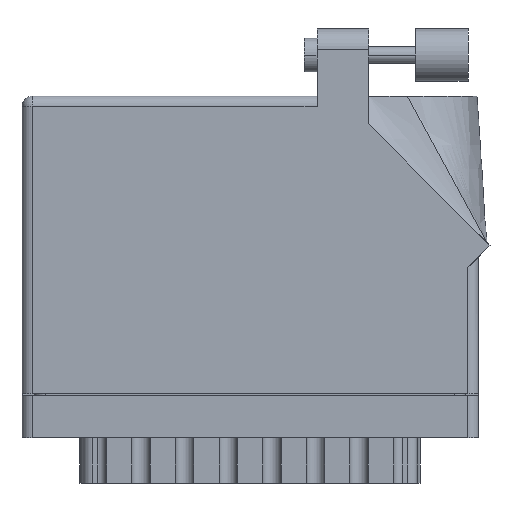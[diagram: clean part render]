
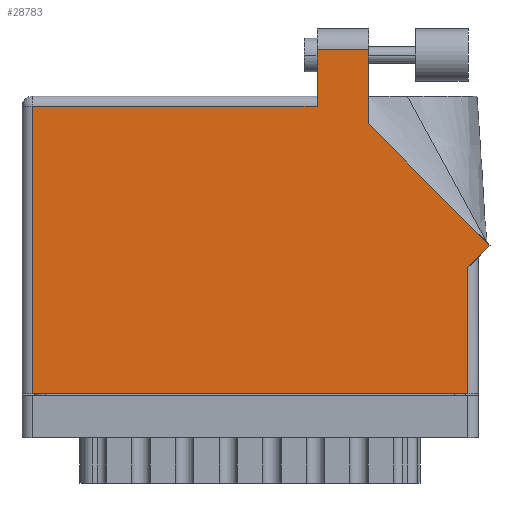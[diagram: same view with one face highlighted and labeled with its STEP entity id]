
A CAD part, front view. The second image highlights one B-rep face of the part: STEP entity #28783.
In plain terms, the highlighted face is planar.
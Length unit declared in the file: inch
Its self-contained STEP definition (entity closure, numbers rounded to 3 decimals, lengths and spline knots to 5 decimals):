
#1003 = DIRECTION ( 'NONE',  ( 0.707, 0.707, 0. ) ) ;
#2508 = ORIENTED_EDGE ( 'NONE', *, *, #10606, .T. ) ;
#4275 = CARTESIAN_POINT ( 'NONE',  ( 2.78871, 0.88571, 0. ) ) ;
#4432 = LINE ( 'NONE', #39975, #25577 ) ;
#4710 = VECTOR ( 'NONE', #21196, 39.37008 ) ;
#4968 = DIRECTION ( 'NONE',  ( 0., -1., 0. ) ) ;
#5135 = LINE ( 'NONE', #36905, #26316 ) ;
#5680 = ORIENTED_EDGE ( 'NONE', *, *, #43925, .T. ) ;
#6126 = LINE ( 'NONE', #54887, #30542 ) ;
#8485 = VERTEX_POINT ( 'NONE', #66346 ) ;
#8774 = LINE ( 'NONE', #14644, #66543 ) ;
#9948 = EDGE_CURVE ( 'NONE', #45223, #14900, #4432, .T. ) ;
#10449 = LINE ( 'NONE', #15242, #34849 ) ;
#10606 = EDGE_CURVE ( 'NONE', #60431, #51326, #5135, .T. ) ;
#11034 = CARTESIAN_POINT ( 'NONE',  ( 2.718, 0.815, 0. ) ) ;
#14378 = LINE ( 'NONE', #4275, #53429 ) ;
#14506 = LINE ( 'NONE', #11034, #49414 ) ;
#14644 = CARTESIAN_POINT ( 'NONE',  ( 2.656, 0.815, 0. ) ) ;
#14900 = VERTEX_POINT ( 'NONE', #62461 ) ;
#15081 = VECTOR ( 'NONE', #45955, 39.37008 ) ;
#15198 = DIRECTION ( 'NONE',  ( 0., 0., -1. ) ) ;
#15242 = CARTESIAN_POINT ( 'NONE',  ( 1.758, 1.775, 0. ) ) ;
#15254 = EDGE_LOOP ( 'NONE', ( #42660, #59265, #28161, #42583, #2508, #37288, #5680, #33372, #50235 ) ) ;
#15649 = EDGE_CURVE ( 'NONE', #51323, #59387, #14506, .T. ) ;
#17108 = EDGE_CURVE ( 'NONE', #51326, #8485, #26468, .T. ) ;
#18757 = CARTESIAN_POINT ( 'NONE',  ( 2.656, 0.753, 0. ) ) ;
#21196 = DIRECTION ( 'NONE',  ( 0., 1., 0. ) ) ;
#22940 = VERTEX_POINT ( 'NONE', #36296 ) ;
#23901 = EDGE_CURVE ( 'NONE', #14900, #54092, #10449, .T. ) ;
#25178 = DIRECTION ( 'NONE',  ( -1., 0., 0. ) ) ;
#25197 = DIRECTION ( 'NONE',  ( -0.707, 0.707, 0. ) ) ;
#25412 = PLANE ( 'NONE',  #38828 ) ;
#25577 = VECTOR ( 'NONE', #36327, 39.37008 ) ;
#26316 = VECTOR ( 'NONE', #58099, 39.37008 ) ;
#26468 = LINE ( 'NONE', #40955, #15081 ) ;
#26677 = CARTESIAN_POINT ( 'NONE',  ( 2.065, 1.60942, 0. ) ) ;
#28161 = ORIENTED_EDGE ( 'NONE', *, *, #23901, .T. ) ;
#28783 = ADVANCED_FACE ( 'NONE', ( #59992 ), #25412, .F. ) ;
#29410 = EDGE_CURVE ( 'NONE', #59387, #22940, #14378, .T. ) ;
#30542 = VECTOR ( 'NONE', #39836, 39.37008 ) ;
#33372 = ORIENTED_EDGE ( 'NONE', *, *, #15649, .T. ) ;
#34849 = VECTOR ( 'NONE', #4968, 39.37008 ) ;
#35710 = DIRECTION ( 'NONE',  ( 0., 1., 0. ) ) ;
#36296 = CARTESIAN_POINT ( 'NONE',  ( 2.065, 1.60942, 0. ) ) ;
#36327 = DIRECTION ( 'NONE',  ( -1., 0., 0. ) ) ;
#36905 = CARTESIAN_POINT ( 'NONE',  ( 0.062, 0., 0. ) ) ;
#37288 = ORIENTED_EDGE ( 'NONE', *, *, #17108, .T. ) ;
#37952 = CARTESIAN_POINT ( 'NONE',  ( 1.758, 1.713, 0. ) ) ;
#38828 = AXIS2_PLACEMENT_3D ( 'NONE', #66929, #15198, #25178 ) ;
#39836 = DIRECTION ( 'NONE',  ( -1., 0., 0. ) ) ;
#39975 = CARTESIAN_POINT ( 'NONE',  ( 1.758, 2.05, 0. ) ) ;
#40955 = CARTESIAN_POINT ( 'NONE',  ( 0., 0., 0. ) ) ;
#42583 = ORIENTED_EDGE ( 'NONE', *, *, #45388, .T. ) ;
#42660 = ORIENTED_EDGE ( 'NONE', *, *, #67329, .T. ) ;
#43925 = EDGE_CURVE ( 'NONE', #8485, #51323, #8774, .T. ) ;
#45223 = VERTEX_POINT ( 'NONE', #48953 ) ;
#45388 = EDGE_CURVE ( 'NONE', #54092, #60431, #6126, .T. ) ;
#45955 = DIRECTION ( 'NONE',  ( 1., 0., 0. ) ) ;
#48522 = CARTESIAN_POINT ( 'NONE',  ( 2.78871, 0.88571, 0. ) ) ;
#48953 = CARTESIAN_POINT ( 'NONE',  ( 2.065, 2.05, 0. ) ) ;
#49414 = VECTOR ( 'NONE', #1003, 39.37008 ) ;
#50235 = ORIENTED_EDGE ( 'NONE', *, *, #29410, .T. ) ;
#51323 = VERTEX_POINT ( 'NONE', #18757 ) ;
#51326 = VERTEX_POINT ( 'NONE', #66227 ) ;
#53429 = VECTOR ( 'NONE', #25197, 39.37008 ) ;
#54092 = VERTEX_POINT ( 'NONE', #37952 ) ;
#54887 = CARTESIAN_POINT ( 'NONE',  ( 0., 1.713, 0. ) ) ;
#56705 = CARTESIAN_POINT ( 'NONE',  ( 0.062, 1.713, 0. ) ) ;
#58099 = DIRECTION ( 'NONE',  ( 0., -1., 0. ) ) ;
#59265 = ORIENTED_EDGE ( 'NONE', *, *, #9948, .T. ) ;
#59387 = VERTEX_POINT ( 'NONE', #48522 ) ;
#59992 = FACE_OUTER_BOUND ( 'NONE', #15254, .T. ) ;
#60431 = VERTEX_POINT ( 'NONE', #56705 ) ;
#62461 = CARTESIAN_POINT ( 'NONE',  ( 1.758, 2.05, 0. ) ) ;
#66227 = CARTESIAN_POINT ( 'NONE',  ( 0.062, 0., 0. ) ) ;
#66346 = CARTESIAN_POINT ( 'NONE',  ( 2.656, 0., 0. ) ) ;
#66509 = LINE ( 'NONE', #26677, #4710 ) ;
#66543 = VECTOR ( 'NONE', #35710, 39.37008 ) ;
#66929 = CARTESIAN_POINT ( 'NONE',  ( 0., 1.775, 0. ) ) ;
#67329 = EDGE_CURVE ( 'NONE', #22940, #45223, #66509, .T. ) ;
